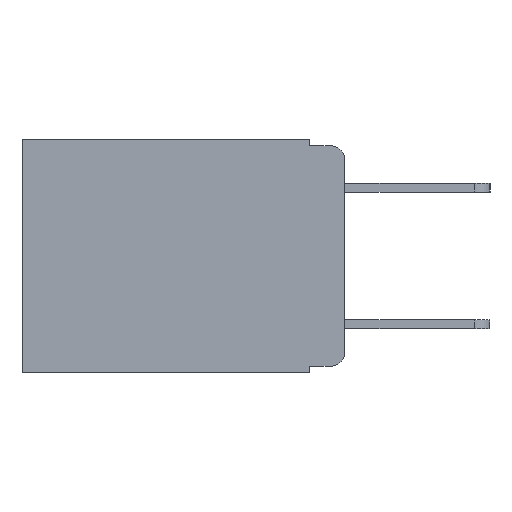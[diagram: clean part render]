
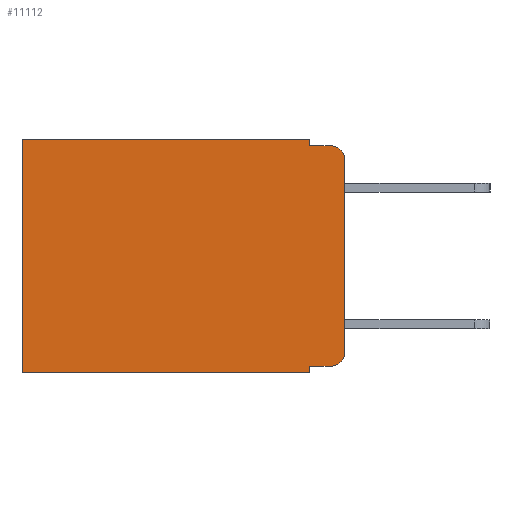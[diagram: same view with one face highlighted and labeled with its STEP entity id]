
A CAD part, left-side view. The second image highlights one B-rep face of the part: STEP entity #11112.
In plain terms, the highlighted planar face has unit normal (-1, 0, 0).
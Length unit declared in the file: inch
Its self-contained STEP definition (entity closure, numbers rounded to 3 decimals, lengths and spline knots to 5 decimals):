
#365 = CARTESIAN_POINT ( 'NONE',  ( 0.298, 0., 0. ) ) ;
#471 = CARTESIAN_POINT ( 'NONE',  ( 0.298, 0.051, -0.343 ) ) ;
#1155 = CARTESIAN_POINT ( 'NONE',  ( 0.298, 0.051, -0.01 ) ) ;
#1177 = VECTOR ( 'NONE', #2293, 39.37008 ) ;
#1299 = DIRECTION ( 'NONE',  ( 0., 0., -1. ) ) ;
#1416 = LINE ( 'NONE', #19836, #14652 ) ;
#1430 = VECTOR ( 'NONE', #2121, 39.37008 ) ;
#1531 = EDGE_CURVE ( 'NONE', #18792, #14813, #17565, .T. ) ;
#2121 = DIRECTION ( 'NONE',  ( 0., 0., -1. ) ) ;
#2293 = DIRECTION ( 'NONE',  ( 0., 0., -1. ) ) ;
#2812 = LINE ( 'NONE', #11335, #11138 ) ;
#3010 = ORIENTED_EDGE ( 'NONE', *, *, #20548, .F. ) ;
#3075 = EDGE_CURVE ( 'NONE', #5464, #18792, #6178, .T. ) ;
#4256 = DIRECTION ( 'NONE',  ( -1., 0., 0. ) ) ;
#4294 = ORIENTED_EDGE ( 'NONE', *, *, #3075, .F. ) ;
#4398 = EDGE_CURVE ( 'NONE', #5464, #21124, #1416, .T. ) ;
#4985 = ORIENTED_EDGE ( 'NONE', *, *, #11291, .T. ) ;
#5080 = VERTEX_POINT ( 'NONE', #21223 ) ;
#5212 = LINE ( 'NONE', #9627, #13499 ) ;
#5280 = CARTESIAN_POINT ( 'NONE',  ( 0.298, 0.02, -0.313 ) ) ;
#5284 = CARTESIAN_POINT ( 'NONE',  ( 0.298, 0.051, -0.01 ) ) ;
#5464 = VERTEX_POINT ( 'NONE', #15146 ) ;
#5892 = LINE ( 'NONE', #10362, #1430 ) ;
#5908 = DIRECTION ( 'NONE',  ( 0., -1., 0. ) ) ;
#6163 = EDGE_CURVE ( 'NONE', #19108, #15392, #16120, .T. ) ;
#6178 = LINE ( 'NONE', #17688, #1177 ) ;
#6860 = EDGE_CURVE ( 'NONE', #15700, #19967, #5892, .T. ) ;
#6995 = DIRECTION ( 'NONE',  ( 0., 0., -1. ) ) ;
#7032 = ORIENTED_EDGE ( 'NONE', *, *, #16270, .T. ) ;
#7640 = ORIENTED_EDGE ( 'NONE', *, *, #12676, .F. ) ;
#8318 = VECTOR ( 'NONE', #5908, 39.37008 ) ;
#8578 = LINE ( 'NONE', #13878, #16308 ) ;
#8804 = AXIS2_PLACEMENT_3D ( 'NONE', #14198, #4256, #15842 ) ;
#8921 = CARTESIAN_POINT ( 'NONE',  ( 0.298, 0.02, -0.01 ) ) ;
#9461 = ORIENTED_EDGE ( 'NONE', *, *, #19343, .T. ) ;
#9627 = CARTESIAN_POINT ( 'NONE',  ( 0.298, 0.051, -0.333 ) ) ;
#9647 = CARTESIAN_POINT ( 'NONE',  ( 0.298, 0., 0. ) ) ;
#10362 = CARTESIAN_POINT ( 'NONE',  ( 0.298, 0.051, 0. ) ) ;
#10375 = DIRECTION ( 'NONE',  ( 0., 0., -1. ) ) ;
#10640 = VECTOR ( 'NONE', #10375, 39.37008 ) ;
#10745 = CIRCLE ( 'NONE', #8804, 0.02 ) ;
#10961 = AXIS2_PLACEMENT_3D ( 'NONE', #5280, #16826, #6995 ) ;
#11112 = ADVANCED_FACE ( 'NONE', ( #19813 ), #19413, .F. ) ;
#11138 = VECTOR ( 'NONE', #19450, 39.37008 ) ;
#11269 = DIRECTION ( 'NONE',  ( 0., -1., 0. ) ) ;
#11291 = EDGE_CURVE ( 'NONE', #21124, #5080, #8578, .T. ) ;
#11292 = DIRECTION ( 'NONE',  ( 1., 0., 0. ) ) ;
#11335 = CARTESIAN_POINT ( 'NONE',  ( 0.298, 0., -0.343 ) ) ;
#12237 = DIRECTION ( 'NONE',  ( 0., 0., -1. ) ) ;
#12676 = EDGE_CURVE ( 'NONE', #19967, #5080, #2812, .T. ) ;
#13499 = VECTOR ( 'NONE', #11269, 39.37008 ) ;
#13618 = DIRECTION ( 'NONE',  ( 0., 1., 0. ) ) ;
#13878 = CARTESIAN_POINT ( 'NONE',  ( 0.298, 0.473, 0. ) ) ;
#14198 = CARTESIAN_POINT ( 'NONE',  ( 0.298, 0.02, -0.03 ) ) ;
#14357 = VERTEX_POINT ( 'NONE', #18807 ) ;
#14414 = ORIENTED_EDGE ( 'NONE', *, *, #4398, .T. ) ;
#14421 = CARTESIAN_POINT ( 'NONE',  ( 0.298, 0.051, -0.333 ) ) ;
#14491 = ORIENTED_EDGE ( 'NONE', *, *, #1531, .F. ) ;
#14596 = ORIENTED_EDGE ( 'NONE', *, *, #6163, .T. ) ;
#14652 = VECTOR ( 'NONE', #13618, 39.37008 ) ;
#14813 = VERTEX_POINT ( 'NONE', #8921 ) ;
#15146 = CARTESIAN_POINT ( 'NONE',  ( 0.298, 0.051, 0. ) ) ;
#15392 = VERTEX_POINT ( 'NONE', #20083 ) ;
#15700 = VERTEX_POINT ( 'NONE', #14421 ) ;
#15842 = DIRECTION ( 'NONE',  ( 0., 0., -1. ) ) ;
#16120 = CIRCLE ( 'NONE', #10961, 0.02 ) ;
#16270 = EDGE_CURVE ( 'NONE', #14357, #14813, #10745, .T. ) ;
#16308 = VECTOR ( 'NONE', #12237, 39.37008 ) ;
#16788 = EDGE_LOOP ( 'NONE', ( #3010, #7032, #14491, #4294, #14414, #4985, #7640, #21239, #9461, #14596 ) ) ;
#16826 = DIRECTION ( 'NONE',  ( -1., 0., 0. ) ) ;
#17235 = CARTESIAN_POINT ( 'NONE',  ( 0.298, 0.02, -0.333 ) ) ;
#17565 = LINE ( 'NONE', #5284, #8318 ) ;
#17688 = CARTESIAN_POINT ( 'NONE',  ( 0.298, 0.051, 0. ) ) ;
#18792 = VERTEX_POINT ( 'NONE', #1155 ) ;
#18807 = CARTESIAN_POINT ( 'NONE',  ( 0.298, 0., -0.03 ) ) ;
#19108 = VERTEX_POINT ( 'NONE', #17235 ) ;
#19313 = LINE ( 'NONE', #365, #10640 ) ;
#19343 = EDGE_CURVE ( 'NONE', #15700, #19108, #5212, .T. ) ;
#19413 = PLANE ( 'NONE',  #20799 ) ;
#19450 = DIRECTION ( 'NONE',  ( 0., 1., 0. ) ) ;
#19813 = FACE_OUTER_BOUND ( 'NONE', #16788, .T. ) ;
#19836 = CARTESIAN_POINT ( 'NONE',  ( 0.298, 0., 0. ) ) ;
#19942 = CARTESIAN_POINT ( 'NONE',  ( 0.298, 0.473, 0. ) ) ;
#19967 = VERTEX_POINT ( 'NONE', #471 ) ;
#20083 = CARTESIAN_POINT ( 'NONE',  ( 0.298, 0., -0.313 ) ) ;
#20548 = EDGE_CURVE ( 'NONE', #14357, #15392, #19313, .T. ) ;
#20799 = AXIS2_PLACEMENT_3D ( 'NONE', #9647, #11292, #1299 ) ;
#21124 = VERTEX_POINT ( 'NONE', #19942 ) ;
#21223 = CARTESIAN_POINT ( 'NONE',  ( 0.298, 0.473, -0.343 ) ) ;
#21239 = ORIENTED_EDGE ( 'NONE', *, *, #6860, .F. ) ;
